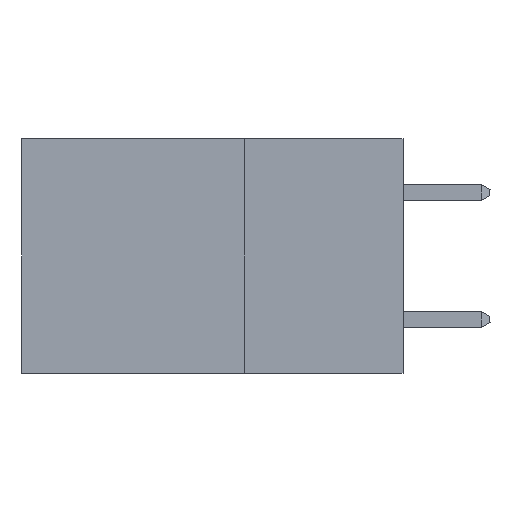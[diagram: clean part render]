
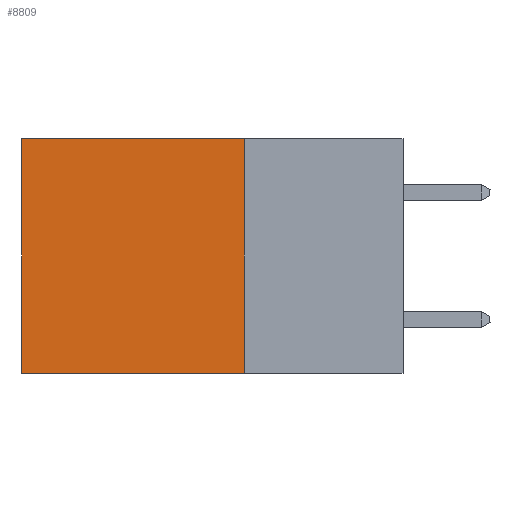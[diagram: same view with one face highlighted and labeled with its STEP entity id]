
A CAD part, left-side view. The second image highlights one B-rep face of the part: STEP entity #8809.
In plain terms, the highlighted planar face has unit normal (-1, 0, 0).
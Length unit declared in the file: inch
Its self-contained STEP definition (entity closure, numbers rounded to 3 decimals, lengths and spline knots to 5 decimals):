
#276 = DIRECTION ( 'NONE',  ( 0., 1., 0. ) ) ;
#1612 = FACE_OUTER_BOUND ( 'NONE', #34775, .T. ) ;
#1782 = ORIENTED_EDGE ( 'NONE', *, *, #25424, .T. ) ;
#2296 = VECTOR ( 'NONE', #27292, 39.37008 ) ;
#2395 = VECTOR ( 'NONE', #276, 39.37008 ) ;
#4188 = CARTESIAN_POINT ( 'NONE',  ( 0.2875, 0.6, 0. ) ) ;
#4413 = CARTESIAN_POINT ( 'NONE',  ( 0.2875, 0.25, 0. ) ) ;
#5791 = EDGE_CURVE ( 'NONE', #29645, #24968, #26244, .T. ) ;
#7336 = DIRECTION ( 'NONE',  ( 0., 0., -1. ) ) ;
#8072 = CARTESIAN_POINT ( 'NONE',  ( 0.2875, 0.6, 0. ) ) ;
#8379 = VERTEX_POINT ( 'NONE', #4188 ) ;
#8809 = ADVANCED_FACE ( 'NONE', ( #1612 ), #27823, .F. ) ;
#9921 = ORIENTED_EDGE ( 'NONE', *, *, #12371, .F. ) ;
#10170 = DIRECTION ( 'NONE',  ( 0., 0., -1. ) ) ;
#12371 = EDGE_CURVE ( 'NONE', #24968, #41076, #30578, .T. ) ;
#13570 = CARTESIAN_POINT ( 'NONE',  ( 0.2875, 0.25, 0. ) ) ;
#15487 = AXIS2_PLACEMENT_3D ( 'NONE', #13570, #31370, #10170 ) ;
#18897 = LINE ( 'NONE', #8072, #44972 ) ;
#20153 = CARTESIAN_POINT ( 'NONE',  ( 0.2875, 0.25, 0. ) ) ;
#21440 = CARTESIAN_POINT ( 'NONE',  ( 0.2875, 0.6, -0.37 ) ) ;
#22686 = ORIENTED_EDGE ( 'NONE', *, *, #5791, .F. ) ;
#24968 = VERTEX_POINT ( 'NONE', #31947 ) ;
#25424 = EDGE_CURVE ( 'NONE', #29645, #8379, #30487, .T. ) ;
#26244 = LINE ( 'NONE', #42627, #34515 ) ;
#27292 = DIRECTION ( 'NONE',  ( 0., 1., 0. ) ) ;
#27823 = PLANE ( 'NONE',  #15487 ) ;
#28590 = CARTESIAN_POINT ( 'NONE',  ( 0.2875, 0.25, -0.37 ) ) ;
#29645 = VERTEX_POINT ( 'NONE', #4413 ) ;
#30487 = LINE ( 'NONE', #20153, #2296 ) ;
#30578 = LINE ( 'NONE', #28590, #2395 ) ;
#30700 = ORIENTED_EDGE ( 'NONE', *, *, #41870, .T. ) ;
#31370 = DIRECTION ( 'NONE',  ( 1., 0., 0. ) ) ;
#31947 = CARTESIAN_POINT ( 'NONE',  ( 0.2875, 0.25, -0.37 ) ) ;
#34515 = VECTOR ( 'NONE', #7336, 39.37008 ) ;
#34775 = EDGE_LOOP ( 'NONE', ( #30700, #9921, #22686, #1782 ) ) ;
#36220 = DIRECTION ( 'NONE',  ( 0., 0., -1. ) ) ;
#41076 = VERTEX_POINT ( 'NONE', #21440 ) ;
#41870 = EDGE_CURVE ( 'NONE', #8379, #41076, #18897, .T. ) ;
#42627 = CARTESIAN_POINT ( 'NONE',  ( 0.2875, 0.25, 0. ) ) ;
#44972 = VECTOR ( 'NONE', #36220, 39.37008 ) ;
